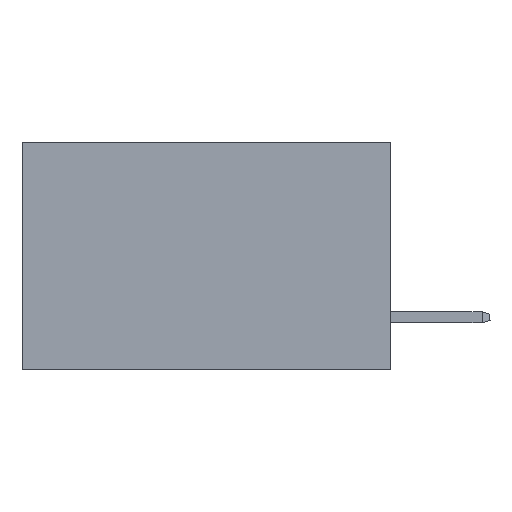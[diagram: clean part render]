
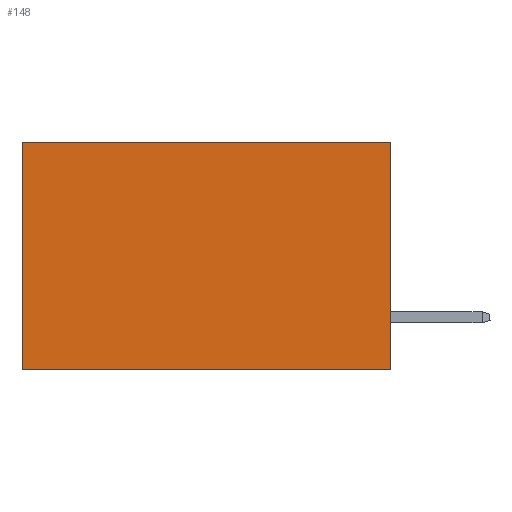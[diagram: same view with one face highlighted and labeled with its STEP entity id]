
A CAD part, left-side view. The second image highlights one B-rep face of the part: STEP entity #148.
In plain terms, the highlighted planar face has unit normal (-1, 0, 0).
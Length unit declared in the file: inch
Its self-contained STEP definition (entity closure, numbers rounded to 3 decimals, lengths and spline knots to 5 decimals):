
#148 = ADVANCED_FACE ( 'NONE', ( #9631 ), #13207, .F. ) ;
#1139 = LINE ( 'NONE', #11085, #10644 ) ;
#1669 = EDGE_CURVE ( 'NONE', #12908, #3872, #13602, .T. ) ;
#2049 = EDGE_CURVE ( 'NONE', #12600, #3872, #13904, .T. ) ;
#2419 = EDGE_LOOP ( 'NONE', ( #13105, #3412, #8235, #13901 ) ) ;
#2976 = EDGE_CURVE ( 'NONE', #11725, #12908, #1139, .T. ) ;
#3246 = DIRECTION ( 'NONE',  ( 0., 0., -1. ) ) ;
#3408 = DIRECTION ( 'NONE',  ( 0., 0., -1. ) ) ;
#3412 = ORIENTED_EDGE ( 'NONE', *, *, #2049, .F. ) ;
#3872 = VERTEX_POINT ( 'NONE', #12067 ) ;
#4009 = VECTOR ( 'NONE', #3408, 39.37008 ) ;
#5302 = CARTESIAN_POINT ( 'NONE',  ( 0.2875, 0.6, 0. ) ) ;
#6124 = CARTESIAN_POINT ( 'NONE',  ( 0.2875, 0., 0. ) ) ;
#7409 = DIRECTION ( 'NONE',  ( 0., 0., -1. ) ) ;
#7463 = LINE ( 'NONE', #9535, #13267 ) ;
#7956 = DIRECTION ( 'NONE',  ( 0., 1., 0. ) ) ;
#8235 = ORIENTED_EDGE ( 'NONE', *, *, #9104, .F. ) ;
#8481 = CARTESIAN_POINT ( 'NONE',  ( 0.2875, 0., -0.37 ) ) ;
#9104 = EDGE_CURVE ( 'NONE', #11725, #12600, #7463, .T. ) ;
#9535 = CARTESIAN_POINT ( 'NONE',  ( 0.2875, 0., 0. ) ) ;
#9631 = FACE_OUTER_BOUND ( 'NONE', #2419, .T. ) ;
#10644 = VECTOR ( 'NONE', #7956, 39.37008 ) ;
#10830 = CARTESIAN_POINT ( 'NONE',  ( 0.2875, 0., -0.37 ) ) ;
#11043 = VECTOR ( 'NONE', #11295, 39.37008 ) ;
#11085 = CARTESIAN_POINT ( 'NONE',  ( 0.2875, 0., 0. ) ) ;
#11295 = DIRECTION ( 'NONE',  ( 0., 1., 0. ) ) ;
#11725 = VERTEX_POINT ( 'NONE', #12659 ) ;
#12067 = CARTESIAN_POINT ( 'NONE',  ( 0.2875, 0.6, -0.37 ) ) ;
#12495 = AXIS2_PLACEMENT_3D ( 'NONE', #6124, #14223, #7409 ) ;
#12600 = VERTEX_POINT ( 'NONE', #10830 ) ;
#12659 = CARTESIAN_POINT ( 'NONE',  ( 0.2875, 0., 0. ) ) ;
#12908 = VERTEX_POINT ( 'NONE', #5302 ) ;
#13105 = ORIENTED_EDGE ( 'NONE', *, *, #1669, .T. ) ;
#13207 = PLANE ( 'NONE',  #12495 ) ;
#13267 = VECTOR ( 'NONE', #3246, 39.37008 ) ;
#13602 = LINE ( 'NONE', #15331, #4009 ) ;
#13901 = ORIENTED_EDGE ( 'NONE', *, *, #2976, .T. ) ;
#13904 = LINE ( 'NONE', #8481, #11043 ) ;
#14223 = DIRECTION ( 'NONE',  ( 1., 0., 0. ) ) ;
#15331 = CARTESIAN_POINT ( 'NONE',  ( 0.2875, 0.6, 0. ) ) ;
